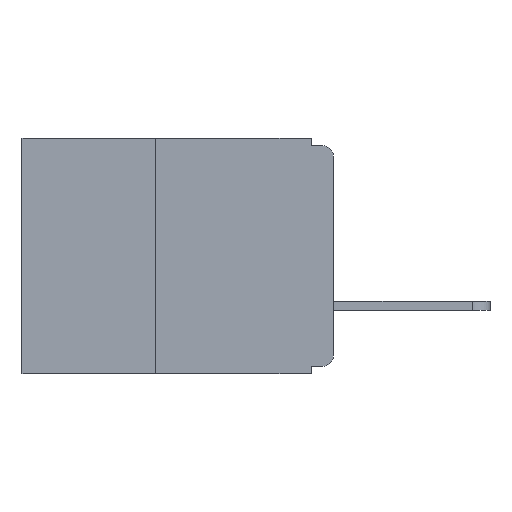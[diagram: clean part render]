
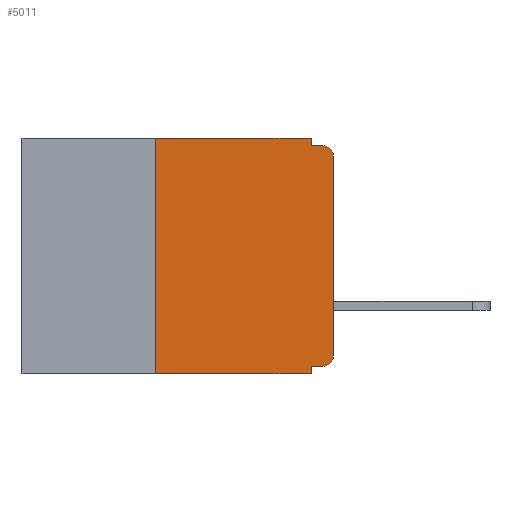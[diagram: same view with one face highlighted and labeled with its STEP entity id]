
A CAD part, left-side view. The second image highlights one B-rep face of the part: STEP entity #5011.
In plain terms, the highlighted planar face has unit normal (-1, 0, 0).
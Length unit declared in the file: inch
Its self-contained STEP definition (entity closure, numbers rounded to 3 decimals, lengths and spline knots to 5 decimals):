
#647 = DIRECTION ( 'NONE',  ( 0., -1., 0. ) ) ;
#990 = CARTESIAN_POINT ( 'NONE',  ( 0., 0.015, -0.01 ) ) ;
#1011 = CARTESIAN_POINT ( 'NONE',  ( 0., 0.437, 0. ) ) ;
#1278 = VECTOR ( 'NONE', #18216, 39.37008 ) ;
#1378 = VECTOR ( 'NONE', #27412, 39.37008 ) ;
#1507 = CARTESIAN_POINT ( 'NONE',  ( 0., 0.25, -0.33 ) ) ;
#2441 = CARTESIAN_POINT ( 'NONE',  ( 0., 0., -0.305 ) ) ;
#3034 = CARTESIAN_POINT ( 'NONE',  ( 0., 0., -0.32 ) ) ;
#3170 = DIRECTION ( 'NONE',  ( -1., 0., 0. ) ) ;
#3459 = VECTOR ( 'NONE', #5115, 39.37008 ) ;
#4237 = EDGE_CURVE ( 'NONE', #27439, #14952, #15851, .T. ) ;
#4484 = EDGE_CURVE ( 'NONE', #20687, #26541, #21380, .T. ) ;
#4675 = PLANE ( 'NONE',  #6845 ) ;
#5011 = ADVANCED_FACE ( 'NONE', ( #7438 ), #4675, .F. ) ;
#5115 = DIRECTION ( 'NONE',  ( 0., 0., -1. ) ) ;
#5468 = ORIENTED_EDGE ( 'NONE', *, *, #4484, .T. ) ;
#5631 = VERTEX_POINT ( 'NONE', #2441 ) ;
#6529 = VECTOR ( 'NONE', #16510, 39.37008 ) ;
#6845 = AXIS2_PLACEMENT_3D ( 'NONE', #13516, #20193, #6898 ) ;
#6898 = DIRECTION ( 'NONE',  ( 0., 0., -1. ) ) ;
#6938 = LINE ( 'NONE', #3034, #23245 ) ;
#7049 = CARTESIAN_POINT ( 'NONE',  ( 0., 0., 0. ) ) ;
#7143 = CARTESIAN_POINT ( 'NONE',  ( 0., 0.25, 0. ) ) ;
#7197 = CIRCLE ( 'NONE', #24198, 0.015 ) ;
#7204 = CARTESIAN_POINT ( 'NONE',  ( 0., 0.437, -0.33 ) ) ;
#7438 = FACE_OUTER_BOUND ( 'NONE', #28638, .T. ) ;
#7565 = CARTESIAN_POINT ( 'NONE',  ( 0., 0., -0.01 ) ) ;
#8195 = CARTESIAN_POINT ( 'NONE',  ( 0., 0., -0.025 ) ) ;
#8703 = VERTEX_POINT ( 'NONE', #24698 ) ;
#8762 = CARTESIAN_POINT ( 'NONE',  ( 0., 0.031, -0.33 ) ) ;
#9357 = LINE ( 'NONE', #18328, #3459 ) ;
#9583 = VECTOR ( 'NONE', #647, 39.37008 ) ;
#9589 = CARTESIAN_POINT ( 'NONE',  ( 0., 0.031, 0. ) ) ;
#9838 = EDGE_CURVE ( 'NONE', #20687, #10995, #19763, .T. ) ;
#10995 = VERTEX_POINT ( 'NONE', #7143 ) ;
#11631 = EDGE_CURVE ( 'NONE', #23885, #12547, #21371, .T. ) ;
#11686 = ORIENTED_EDGE ( 'NONE', *, *, #24345, .T. ) ;
#12059 = CARTESIAN_POINT ( 'NONE',  ( 0., 0.015, -0.305 ) ) ;
#12547 = VERTEX_POINT ( 'NONE', #990 ) ;
#12679 = CARTESIAN_POINT ( 'NONE',  ( 0., 0.031, 0. ) ) ;
#12871 = VECTOR ( 'NONE', #27574, 39.37008 ) ;
#12966 = ORIENTED_EDGE ( 'NONE', *, *, #11631, .T. ) ;
#13516 = CARTESIAN_POINT ( 'NONE',  ( 0., 0.437, 0. ) ) ;
#14278 = DIRECTION ( 'NONE',  ( 0., 0., -1. ) ) ;
#14825 = EDGE_CURVE ( 'NONE', #5631, #23885, #24183, .T. ) ;
#14901 = DIRECTION ( 'NONE',  ( 0., 0., -1. ) ) ;
#14952 = VERTEX_POINT ( 'NONE', #19169 ) ;
#15099 = ORIENTED_EDGE ( 'NONE', *, *, #9838, .F. ) ;
#15851 = LINE ( 'NONE', #12679, #26963 ) ;
#16341 = CARTESIAN_POINT ( 'NONE',  ( 0., 0.25, -0.33 ) ) ;
#16442 = CARTESIAN_POINT ( 'NONE',  ( 0., 0.015, -0.025 ) ) ;
#16510 = DIRECTION ( 'NONE',  ( 0., -1., 0. ) ) ;
#18216 = DIRECTION ( 'NONE',  ( 0., 0., 1. ) ) ;
#18324 = LINE ( 'NONE', #1011, #6529 ) ;
#18328 = CARTESIAN_POINT ( 'NONE',  ( 0., 0.031, -0.33 ) ) ;
#18666 = DIRECTION ( 'NONE',  ( 0., 0., -1. ) ) ;
#18746 = LINE ( 'NONE', #7565, #12871 ) ;
#19169 = CARTESIAN_POINT ( 'NONE',  ( 0., 0.031, -0.01 ) ) ;
#19687 = CARTESIAN_POINT ( 'NONE',  ( 0., 0.015, -0.32 ) ) ;
#19763 = LINE ( 'NONE', #16341, #1378 ) ;
#20193 = DIRECTION ( 'NONE',  ( 1., 0., 0. ) ) ;
#20550 = EDGE_CURVE ( 'NONE', #14952, #12547, #18746, .T. ) ;
#20687 = VERTEX_POINT ( 'NONE', #1507 ) ;
#20750 = DIRECTION ( 'NONE',  ( 0., 1., 0. ) ) ;
#21116 = EDGE_CURVE ( 'NONE', #8703, #26541, #9357, .T. ) ;
#21355 = VERTEX_POINT ( 'NONE', #19687 ) ;
#21371 = CIRCLE ( 'NONE', #25507, 0.015 ) ;
#21380 = LINE ( 'NONE', #7204, #9583 ) ;
#23245 = VECTOR ( 'NONE', #20750, 39.37008 ) ;
#23885 = VERTEX_POINT ( 'NONE', #8195 ) ;
#24183 = LINE ( 'NONE', #7049, #1278 ) ;
#24198 = AXIS2_PLACEMENT_3D ( 'NONE', #12059, #27576, #14278 ) ;
#24345 = EDGE_CURVE ( 'NONE', #21355, #5631, #7197, .T. ) ;
#24361 = EDGE_CURVE ( 'NONE', #10995, #27439, #18324, .T. ) ;
#24698 = CARTESIAN_POINT ( 'NONE',  ( 0., 0.031, -0.32 ) ) ;
#25308 = ORIENTED_EDGE ( 'NONE', *, *, #20550, .F. ) ;
#25507 = AXIS2_PLACEMENT_3D ( 'NONE', #16442, #3170, #18666 ) ;
#25620 = ORIENTED_EDGE ( 'NONE', *, *, #24361, .F. ) ;
#26090 = ORIENTED_EDGE ( 'NONE', *, *, #21116, .F. ) ;
#26541 = VERTEX_POINT ( 'NONE', #8762 ) ;
#26676 = ORIENTED_EDGE ( 'NONE', *, *, #28665, .F. ) ;
#26963 = VECTOR ( 'NONE', #14901, 39.37008 ) ;
#27214 = ORIENTED_EDGE ( 'NONE', *, *, #4237, .F. ) ;
#27337 = ORIENTED_EDGE ( 'NONE', *, *, #14825, .T. ) ;
#27412 = DIRECTION ( 'NONE',  ( 0., 0., 1. ) ) ;
#27439 = VERTEX_POINT ( 'NONE', #9589 ) ;
#27574 = DIRECTION ( 'NONE',  ( 0., -1., 0. ) ) ;
#27576 = DIRECTION ( 'NONE',  ( -1., 0., 0. ) ) ;
#28638 = EDGE_LOOP ( 'NONE', ( #27337, #12966, #25308, #27214, #25620, #15099, #5468, #26090, #26676, #11686 ) ) ;
#28665 = EDGE_CURVE ( 'NONE', #21355, #8703, #6938, .T. ) ;
